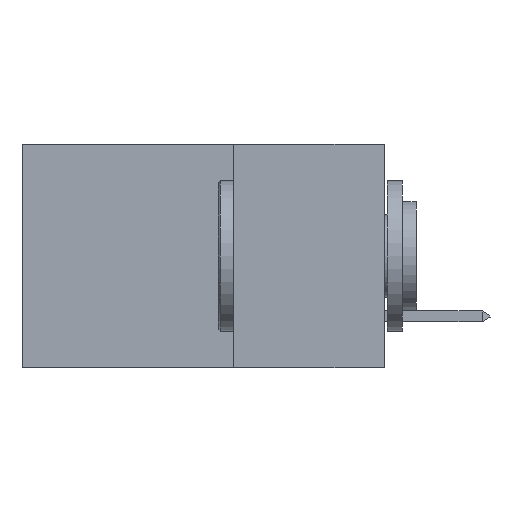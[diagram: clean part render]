
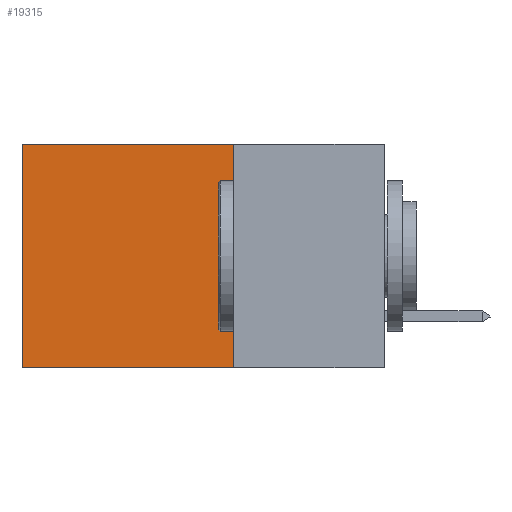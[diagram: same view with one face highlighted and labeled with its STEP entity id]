
A CAD part, left-side view. The second image highlights one B-rep face of the part: STEP entity #19315.
In plain terms, the highlighted planar face has unit normal (-1, 0, 0).
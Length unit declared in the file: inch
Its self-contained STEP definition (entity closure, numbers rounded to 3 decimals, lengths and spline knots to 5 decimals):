
#2886 = CARTESIAN_POINT ( 'NONE',  ( 0.2875, 0.25, 0. ) ) ;
#2938 = VERTEX_POINT ( 'NONE', #30496 ) ;
#3273 = LINE ( 'NONE', #35799, #37045 ) ;
#3676 = EDGE_LOOP ( 'NONE', ( #25806, #13286, #18020, #47788 ) ) ;
#4812 = EDGE_CURVE ( 'NONE', #17710, #20828, #3273, .T. ) ;
#7001 = FACE_OUTER_BOUND ( 'NONE', #3676, .T. ) ;
#8822 = CARTESIAN_POINT ( 'NONE',  ( 0.2875, 0.25, -0.37 ) ) ;
#9750 = CARTESIAN_POINT ( 'NONE',  ( 0.2875, 0.6, 0. ) ) ;
#10230 = DIRECTION ( 'NONE',  ( 0., 0., -1. ) ) ;
#10419 = EDGE_CURVE ( 'NONE', #2938, #38073, #47212, .T. ) ;
#13286 = ORIENTED_EDGE ( 'NONE', *, *, #10419, .F. ) ;
#16116 = EDGE_CURVE ( 'NONE', #20828, #38073, #19101, .T. ) ;
#16922 = DIRECTION ( 'NONE',  ( 0., 1., 0. ) ) ;
#17710 = VERTEX_POINT ( 'NONE', #30300 ) ;
#18020 = ORIENTED_EDGE ( 'NONE', *, *, #41366, .F. ) ;
#19101 = LINE ( 'NONE', #9750, #48783 ) ;
#19315 = ADVANCED_FACE ( 'NONE', ( #7001 ), #48329, .F. ) ;
#20828 = VERTEX_POINT ( 'NONE', #44479 ) ;
#25184 = VECTOR ( 'NONE', #46147, 39.37008 ) ;
#25806 = ORIENTED_EDGE ( 'NONE', *, *, #16116, .T. ) ;
#26031 = DIRECTION ( 'NONE',  ( 1., 0., 0. ) ) ;
#29827 = DIRECTION ( 'NONE',  ( 0., 0., -1. ) ) ;
#30300 = CARTESIAN_POINT ( 'NONE',  ( 0.2875, 0.25, 0. ) ) ;
#30496 = CARTESIAN_POINT ( 'NONE',  ( 0.2875, 0.25, -0.37 ) ) ;
#31413 = CARTESIAN_POINT ( 'NONE',  ( 0.2875, 0.6, -0.37 ) ) ;
#35799 = CARTESIAN_POINT ( 'NONE',  ( 0.2875, 0.25, 0. ) ) ;
#37045 = VECTOR ( 'NONE', #16922, 39.37008 ) ;
#38073 = VERTEX_POINT ( 'NONE', #31413 ) ;
#39113 = VECTOR ( 'NONE', #47771, 39.37008 ) ;
#41366 = EDGE_CURVE ( 'NONE', #17710, #2938, #45632, .T. ) ;
#44479 = CARTESIAN_POINT ( 'NONE',  ( 0.2875, 0.6, 0. ) ) ;
#44946 = CARTESIAN_POINT ( 'NONE',  ( 0.2875, 0.25, 0. ) ) ;
#45632 = LINE ( 'NONE', #44946, #39113 ) ;
#45650 = AXIS2_PLACEMENT_3D ( 'NONE', #2886, #26031, #29827 ) ;
#46147 = DIRECTION ( 'NONE',  ( 0., 1., 0. ) ) ;
#47212 = LINE ( 'NONE', #8822, #25184 ) ;
#47771 = DIRECTION ( 'NONE',  ( 0., 0., -1. ) ) ;
#47788 = ORIENTED_EDGE ( 'NONE', *, *, #4812, .T. ) ;
#48329 = PLANE ( 'NONE',  #45650 ) ;
#48783 = VECTOR ( 'NONE', #10230, 39.37008 ) ;
